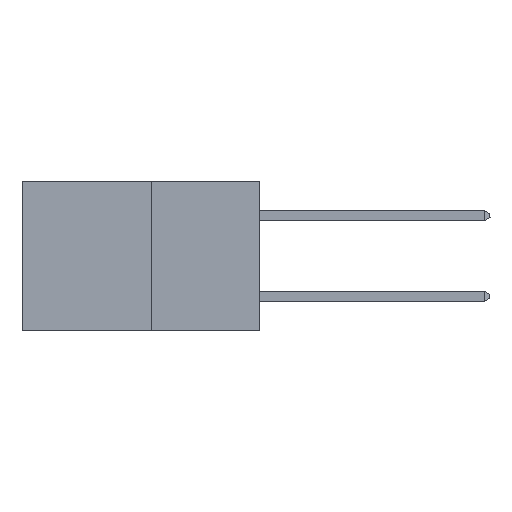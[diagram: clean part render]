
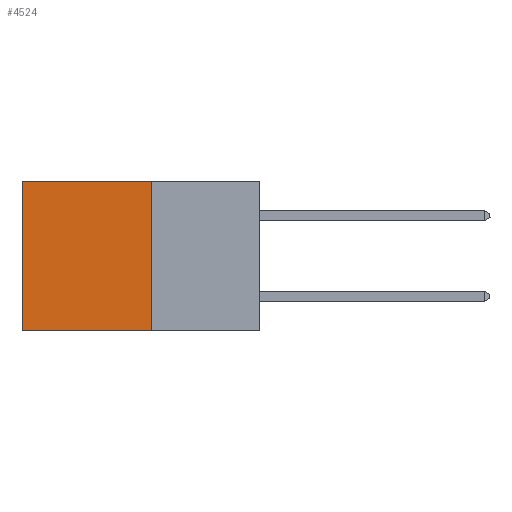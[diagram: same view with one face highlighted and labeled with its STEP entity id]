
A CAD part, left-side view. The second image highlights one B-rep face of the part: STEP entity #4524.
In plain terms, the highlighted planar face has unit normal (-1, 0, 0).
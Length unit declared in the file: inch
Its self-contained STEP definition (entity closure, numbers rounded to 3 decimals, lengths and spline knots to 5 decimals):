
#507 = FACE_OUTER_BOUND ( 'NONE', #3745, .T. ) ;
#1047 = CARTESIAN_POINT ( 'NONE',  ( 0.277, 0.27, -0.37 ) ) ;
#1201 = DIRECTION ( 'NONE',  ( 0., 1., 0. ) ) ;
#1324 = EDGE_CURVE ( 'NONE', #8013, #5296, #8289, .T. ) ;
#1411 = DIRECTION ( 'NONE',  ( 0., 0., -1. ) ) ;
#1468 = CARTESIAN_POINT ( 'NONE',  ( 0.277, 0.27, -0.37 ) ) ;
#1706 = LINE ( 'NONE', #1047, #8887 ) ;
#1768 = DIRECTION ( 'NONE',  ( 0., 1., 0. ) ) ;
#1969 = EDGE_CURVE ( 'NONE', #5296, #4748, #7012, .T. ) ;
#2145 = EDGE_CURVE ( 'NONE', #8174, #4748, #1706, .T. ) ;
#2167 = ORIENTED_EDGE ( 'NONE', *, *, #1969, .T. ) ;
#2219 = CARTESIAN_POINT ( 'NONE',  ( 0.277, 0.59, -0.37 ) ) ;
#2785 = ORIENTED_EDGE ( 'NONE', *, *, #4618, .F. ) ;
#3013 = DIRECTION ( 'NONE',  ( 0., 0., -1. ) ) ;
#3021 = DIRECTION ( 'NONE',  ( 1., 0., 0. ) ) ;
#3031 = PLANE ( 'NONE',  #3926 ) ;
#3173 = VECTOR ( 'NONE', #6479, 39.37008 ) ;
#3190 = CARTESIAN_POINT ( 'NONE',  ( 0.277, 0.27, -0.37 ) ) ;
#3193 = VECTOR ( 'NONE', #1411, 39.37008 ) ;
#3745 = EDGE_LOOP ( 'NONE', ( #2167, #5955, #2785, #4712 ) ) ;
#3926 = AXIS2_PLACEMENT_3D ( 'NONE', #3190, #3021, #3013 ) ;
#4090 = CARTESIAN_POINT ( 'NONE',  ( 0.277, 0.27, -0.37 ) ) ;
#4524 = ADVANCED_FACE ( 'NONE', ( #507 ), #3031, .F. ) ;
#4618 = EDGE_CURVE ( 'NONE', #8013, #8174, #6801, .T. ) ;
#4712 = ORIENTED_EDGE ( 'NONE', *, *, #1324, .T. ) ;
#4748 = VERTEX_POINT ( 'NONE', #6167 ) ;
#5214 = CARTESIAN_POINT ( 'NONE',  ( 0.277, 0.27, 0. ) ) ;
#5296 = VERTEX_POINT ( 'NONE', #5859 ) ;
#5629 = CARTESIAN_POINT ( 'NONE',  ( 0.277, 0.27, 0. ) ) ;
#5859 = CARTESIAN_POINT ( 'NONE',  ( 0.277, 0.59, 0. ) ) ;
#5955 = ORIENTED_EDGE ( 'NONE', *, *, #2145, .F. ) ;
#6167 = CARTESIAN_POINT ( 'NONE',  ( 0.277, 0.59, -0.37 ) ) ;
#6463 = VECTOR ( 'NONE', #1768, 39.37008 ) ;
#6479 = DIRECTION ( 'NONE',  ( 0., 0., -1. ) ) ;
#6801 = LINE ( 'NONE', #1468, #3193 ) ;
#7012 = LINE ( 'NONE', #2219, #3173 ) ;
#8013 = VERTEX_POINT ( 'NONE', #5214 ) ;
#8174 = VERTEX_POINT ( 'NONE', #4090 ) ;
#8289 = LINE ( 'NONE', #5629, #6463 ) ;
#8887 = VECTOR ( 'NONE', #1201, 39.37008 ) ;
